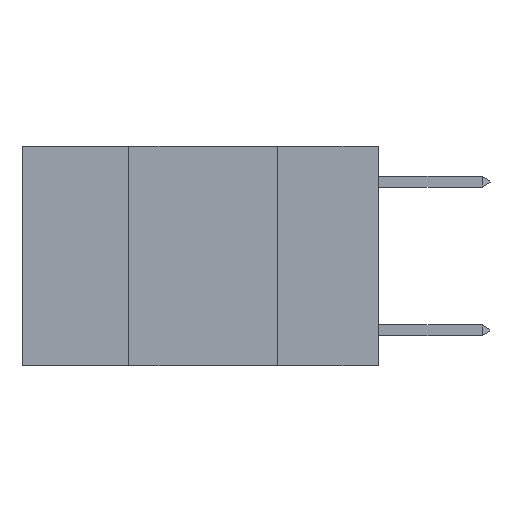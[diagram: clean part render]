
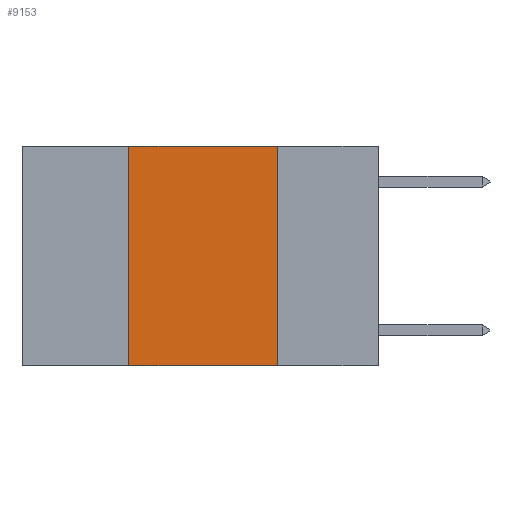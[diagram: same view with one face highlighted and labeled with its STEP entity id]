
A CAD part, left-side view. The second image highlights one B-rep face of the part: STEP entity #9153.
In plain terms, the highlighted planar face has unit normal (-1, 0, 0).
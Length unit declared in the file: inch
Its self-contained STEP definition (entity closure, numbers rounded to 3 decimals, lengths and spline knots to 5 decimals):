
#196 = ORIENTED_EDGE ( 'NONE', *, *, #4613, .F. ) ;
#392 = VECTOR ( 'NONE', #5143, 39.37008 ) ;
#796 = EDGE_LOOP ( 'NONE', ( #9209, #16649, #196, #2917 ) ) ;
#946 = LINE ( 'NONE', #11390, #7919 ) ;
#2048 = AXIS2_PLACEMENT_3D ( 'NONE', #16045, #5946, #7098 ) ;
#2395 = CARTESIAN_POINT ( 'NONE',  ( 0., 0.42, 0. ) ) ;
#2435 = CARTESIAN_POINT ( 'NONE',  ( 0., 0.17, 0. ) ) ;
#2917 = ORIENTED_EDGE ( 'NONE', *, *, #12913, .T. ) ;
#2957 = CARTESIAN_POINT ( 'NONE',  ( 0., 0.42, 0. ) ) ;
#3404 = CARTESIAN_POINT ( 'NONE',  ( 0., 0.6, 0. ) ) ;
#3517 = CARTESIAN_POINT ( 'NONE',  ( 0., 0.17, -0.37 ) ) ;
#3869 = LINE ( 'NONE', #2395, #13247 ) ;
#4432 = DIRECTION ( 'NONE',  ( 0., -1., 0. ) ) ;
#4496 = FACE_OUTER_BOUND ( 'NONE', #796, .T. ) ;
#4613 = EDGE_CURVE ( 'NONE', #14654, #16501, #3869, .T. ) ;
#5143 = DIRECTION ( 'NONE',  ( 0., 0., -1. ) ) ;
#5149 = CARTESIAN_POINT ( 'NONE',  ( 0., 0.17, 0. ) ) ;
#5413 = VERTEX_POINT ( 'NONE', #5149 ) ;
#5946 = DIRECTION ( 'NONE',  ( 1., 0., 0. ) ) ;
#6995 = CARTESIAN_POINT ( 'NONE',  ( 0., 0.42, -0.37 ) ) ;
#7098 = DIRECTION ( 'NONE',  ( 0., 0., -1. ) ) ;
#7919 = VECTOR ( 'NONE', #17214, 39.37008 ) ;
#9153 = ADVANCED_FACE ( 'NONE', ( #4496 ), #13271, .F. ) ;
#9209 = ORIENTED_EDGE ( 'NONE', *, *, #15202, .F. ) ;
#11129 = DIRECTION ( 'NONE',  ( 0., 0., 1. ) ) ;
#11390 = CARTESIAN_POINT ( 'NONE',  ( 0., 0.6, -0.37 ) ) ;
#12487 = LINE ( 'NONE', #2435, #392 ) ;
#12913 = EDGE_CURVE ( 'NONE', #14654, #15465, #946, .T. ) ;
#13247 = VECTOR ( 'NONE', #11129, 39.37008 ) ;
#13271 = PLANE ( 'NONE',  #2048 ) ;
#14654 = VERTEX_POINT ( 'NONE', #6995 ) ;
#15202 = EDGE_CURVE ( 'NONE', #5413, #15465, #12487, .T. ) ;
#15465 = VERTEX_POINT ( 'NONE', #3517 ) ;
#16045 = CARTESIAN_POINT ( 'NONE',  ( 0., 0.6, 0. ) ) ;
#16167 = VECTOR ( 'NONE', #4432, 39.37008 ) ;
#16457 = LINE ( 'NONE', #3404, #16167 ) ;
#16501 = VERTEX_POINT ( 'NONE', #2957 ) ;
#16633 = EDGE_CURVE ( 'NONE', #16501, #5413, #16457, .T. ) ;
#16649 = ORIENTED_EDGE ( 'NONE', *, *, #16633, .F. ) ;
#17214 = DIRECTION ( 'NONE',  ( 0., -1., 0. ) ) ;
